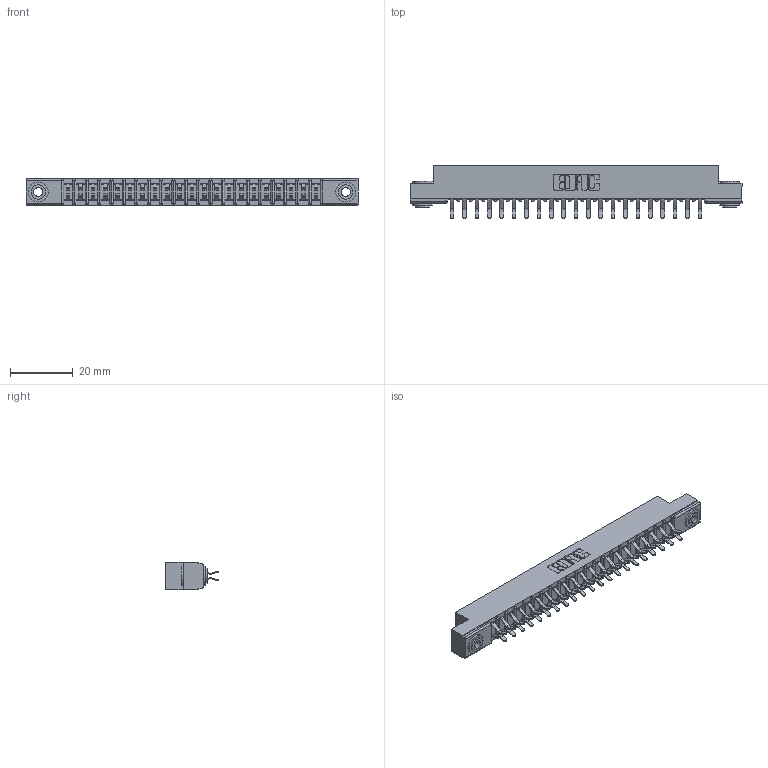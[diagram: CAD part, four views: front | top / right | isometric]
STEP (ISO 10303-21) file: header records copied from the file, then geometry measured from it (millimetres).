
FILE_DESCRIPTION (( 'STEP AP203' ), '1' );
FILE_NAME ('307-042-456-203.STEP', '2020-09-29T23:38:34', ( '' ), ( '' ), 'SwSTEP 2.0', 'SolidWorks 2020', '' );
FILE_SCHEMA (( 'CONFIG_CONTROL_DESIGN' ));
Length unit declared in the file: inch
Products named in the file (4): 345-250-002_345-250-002-102; 307 Part_.156 Dia Mounting Holes; 307-290-001_556; 307-042-456-203
Assembly tree (45 placements, depth 2):
  307-042-456-203
    307 Part_.156 Dia Mounting Holes
    307-290-001_556  x42
    345-250-002_345-250-002-102  x2
Bounding box: 106.22 x 16.97 x 8.71 mm (x, y, z)
Volume: 6941.9 mm3; surface area: 12414.2 mm2
Topology: 45 solids, 45 shells, 2292 faces, 6399 edges, 4146 vertices
Faces by surface type: plane 1480, cylinder 760, sphere 44, cone 8
Entity records: 22433 total; most frequent: CARTESIAN_POINT 3658, ORIENTED_EDGE 3614, DIRECTION 3607, EDGE_CURVE 1807, LINE 1369, VECTOR 1369, VERTEX_POINT 1170, AXIS2_PLACEMENT_3D 1119
